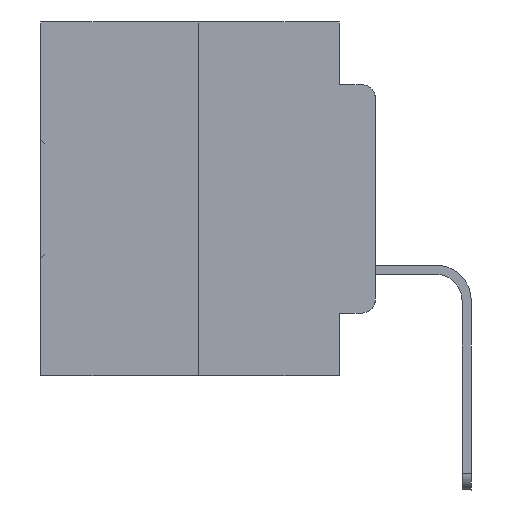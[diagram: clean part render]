
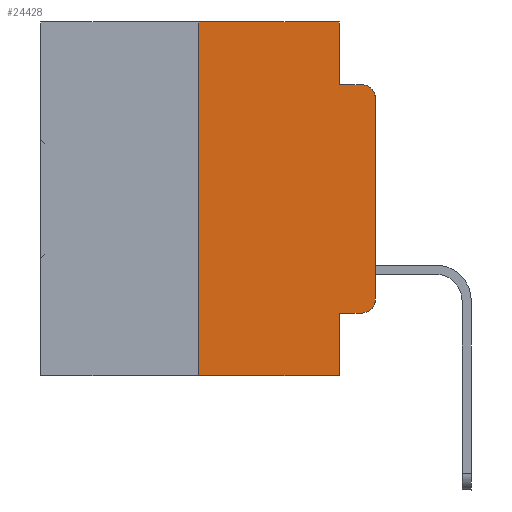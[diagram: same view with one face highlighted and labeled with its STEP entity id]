
A CAD part, left-side view. The second image highlights one B-rep face of the part: STEP entity #24428.
In plain terms, the highlighted planar face has unit normal (-1, 0, 0).
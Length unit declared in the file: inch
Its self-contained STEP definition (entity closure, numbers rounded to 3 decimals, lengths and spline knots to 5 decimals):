
#479 = AXIS2_PLACEMENT_3D ( 'NONE', #20973, #16192, #15847 ) ;
#735 = DIRECTION ( 'NONE',  ( -1., 0., 0. ) ) ;
#1353 = CARTESIAN_POINT ( 'NONE',  ( 0., 0.051, -0.0885 ) ) ;
#1875 = CARTESIAN_POINT ( 'NONE',  ( 0., 0.051, 0. ) ) ;
#2311 = ORIENTED_EDGE ( 'NONE', *, *, #8511, .T. ) ;
#2352 = VECTOR ( 'NONE', #9222, 39.37008 ) ;
#2461 = CARTESIAN_POINT ( 'NONE',  ( 0., 0., -0.1085 ) ) ;
#3513 = CARTESIAN_POINT ( 'NONE',  ( 0., 0.02, -0.3915 ) ) ;
#4099 = ORIENTED_EDGE ( 'NONE', *, *, #11857, .F. ) ;
#5255 = CARTESIAN_POINT ( 'NONE',  ( 0., 0.051, 0. ) ) ;
#6444 = ORIENTED_EDGE ( 'NONE', *, *, #8904, .F. ) ;
#6933 = DIRECTION ( 'NONE',  ( 0., 0., -1. ) ) ;
#7127 = DIRECTION ( 'NONE',  ( 0., 0., 1. ) ) ;
#7364 = LINE ( 'NONE', #12463, #18867 ) ;
#7648 = LINE ( 'NONE', #25091, #18738 ) ;
#7837 = EDGE_CURVE ( 'NONE', #8748, #13949, #8919, .T. ) ;
#8053 = ORIENTED_EDGE ( 'NONE', *, *, #7837, .F. ) ;
#8511 = EDGE_CURVE ( 'NONE', #8748, #31200, #32724, .T. ) ;
#8748 = VERTEX_POINT ( 'NONE', #11657 ) ;
#8904 = EDGE_CURVE ( 'NONE', #26894, #32268, #7648, .T. ) ;
#8919 = LINE ( 'NONE', #5255, #14885 ) ;
#9222 = DIRECTION ( 'NONE',  ( 0., 0., 1. ) ) ;
#9586 = DIRECTION ( 'NONE',  ( -1., 0., 0. ) ) ;
#9918 = CARTESIAN_POINT ( 'NONE',  ( 0., 0.02, -0.0885 ) ) ;
#10499 = VERTEX_POINT ( 'NONE', #10571 ) ;
#10571 = CARTESIAN_POINT ( 'NONE',  ( 0., 0.25, 0. ) ) ;
#11302 = CIRCLE ( 'NONE', #27441, 0.02 ) ;
#11657 = CARTESIAN_POINT ( 'NONE',  ( 0., 0.051, -0.4115 ) ) ;
#11731 = CARTESIAN_POINT ( 'NONE',  ( 0., 0.02, -0.1085 ) ) ;
#11857 = EDGE_CURVE ( 'NONE', #23617, #10499, #31755, .T. ) ;
#12463 = CARTESIAN_POINT ( 'NONE',  ( 0., 0.473, -0.5 ) ) ;
#12494 = VERTEX_POINT ( 'NONE', #1875 ) ;
#13009 = EDGE_CURVE ( 'NONE', #31200, #22441, #23721, .T. ) ;
#13378 = LINE ( 'NONE', #31613, #14168 ) ;
#13949 = VERTEX_POINT ( 'NONE', #29807 ) ;
#14168 = VECTOR ( 'NONE', #31498, 39.37008 ) ;
#14378 = ORIENTED_EDGE ( 'NONE', *, *, #31367, .F. ) ;
#14885 = VECTOR ( 'NONE', #30883, 39.37008 ) ;
#15847 = DIRECTION ( 'NONE',  ( 0., 0., -1. ) ) ;
#16192 = DIRECTION ( 'NONE',  ( 1., 0., 0. ) ) ;
#16204 = LINE ( 'NONE', #29359, #32104 ) ;
#16268 = ORIENTED_EDGE ( 'NONE', *, *, #21440, .T. ) ;
#16659 = CARTESIAN_POINT ( 'NONE',  ( 0., 0.25, 0. ) ) ;
#16735 = VERTEX_POINT ( 'NONE', #2461 ) ;
#17970 = EDGE_LOOP ( 'NONE', ( #27872, #16268, #6444, #29842, #14378, #4099, #30155, #8053, #2311, #27930 ) ) ;
#18716 = CARTESIAN_POINT ( 'NONE',  ( 0., 0., -0.3915 ) ) ;
#18738 = VECTOR ( 'NONE', #32383, 39.37008 ) ;
#18867 = VECTOR ( 'NONE', #19556, 39.37008 ) ;
#19556 = DIRECTION ( 'NONE',  ( 0., -1., 0. ) ) ;
#20276 = EDGE_CURVE ( 'NONE', #23617, #13949, #7364, .T. ) ;
#20309 = VECTOR ( 'NONE', #30838, 39.37008 ) ;
#20973 = CARTESIAN_POINT ( 'NONE',  ( 0., 0.473, 0. ) ) ;
#21127 = LINE ( 'NONE', #25884, #20309 ) ;
#21440 = EDGE_CURVE ( 'NONE', #16735, #32268, #11302, .T. ) ;
#22263 = EDGE_CURVE ( 'NONE', #12494, #26894, #21127, .T. ) ;
#22320 = CARTESIAN_POINT ( 'NONE',  ( 0., 0.02, -0.4115 ) ) ;
#22441 = VERTEX_POINT ( 'NONE', #18716 ) ;
#23617 = VERTEX_POINT ( 'NONE', #24369 ) ;
#23721 = CIRCLE ( 'NONE', #26862, 0.02 ) ;
#23850 = DIRECTION ( 'NONE',  ( 0., 0., -1. ) ) ;
#24369 = CARTESIAN_POINT ( 'NONE',  ( 0., 0.25, -0.5 ) ) ;
#24428 = ADVANCED_FACE ( 'NONE', ( #30420 ), #31169, .F. ) ;
#25091 = CARTESIAN_POINT ( 'NONE',  ( 0., 0.051, -0.0885 ) ) ;
#25674 = CARTESIAN_POINT ( 'NONE',  ( 0., 0.051, -0.4115 ) ) ;
#25884 = CARTESIAN_POINT ( 'NONE',  ( 0., 0.051, 0. ) ) ;
#26862 = AXIS2_PLACEMENT_3D ( 'NONE', #3513, #735, #23850 ) ;
#26894 = VERTEX_POINT ( 'NONE', #1353 ) ;
#27441 = AXIS2_PLACEMENT_3D ( 'NONE', #11731, #9586, #6933 ) ;
#27872 = ORIENTED_EDGE ( 'NONE', *, *, #30413, .T. ) ;
#27930 = ORIENTED_EDGE ( 'NONE', *, *, #13009, .T. ) ;
#28361 = VECTOR ( 'NONE', #30634, 39.37008 ) ;
#29359 = CARTESIAN_POINT ( 'NONE',  ( 0., 0., 0. ) ) ;
#29807 = CARTESIAN_POINT ( 'NONE',  ( 0., 0.051, -0.5 ) ) ;
#29842 = ORIENTED_EDGE ( 'NONE', *, *, #22263, .F. ) ;
#30155 = ORIENTED_EDGE ( 'NONE', *, *, #20276, .T. ) ;
#30413 = EDGE_CURVE ( 'NONE', #22441, #16735, #16204, .T. ) ;
#30420 = FACE_OUTER_BOUND ( 'NONE', #17970, .T. ) ;
#30634 = DIRECTION ( 'NONE',  ( 0., -1., 0. ) ) ;
#30838 = DIRECTION ( 'NONE',  ( 0., 0., -1. ) ) ;
#30883 = DIRECTION ( 'NONE',  ( 0., 0., -1. ) ) ;
#31169 = PLANE ( 'NONE',  #479 ) ;
#31200 = VERTEX_POINT ( 'NONE', #22320 ) ;
#31367 = EDGE_CURVE ( 'NONE', #10499, #12494, #13378, .T. ) ;
#31498 = DIRECTION ( 'NONE',  ( 0., -1., 0. ) ) ;
#31613 = CARTESIAN_POINT ( 'NONE',  ( 0., 0.473, 0. ) ) ;
#31755 = LINE ( 'NONE', #16659, #2352 ) ;
#32104 = VECTOR ( 'NONE', #7127, 39.37008 ) ;
#32268 = VERTEX_POINT ( 'NONE', #9918 ) ;
#32383 = DIRECTION ( 'NONE',  ( 0., -1., 0. ) ) ;
#32724 = LINE ( 'NONE', #25674, #28361 ) ;
